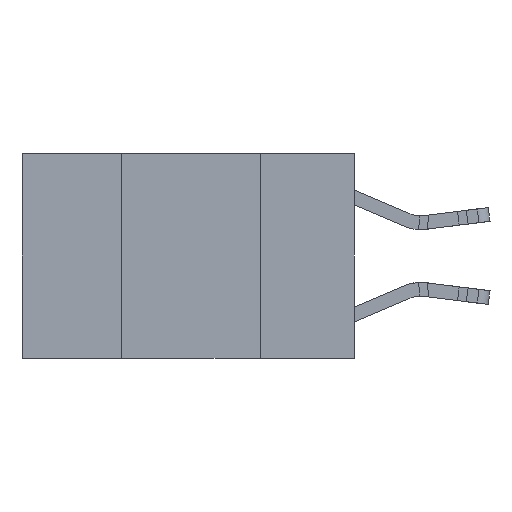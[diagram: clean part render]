
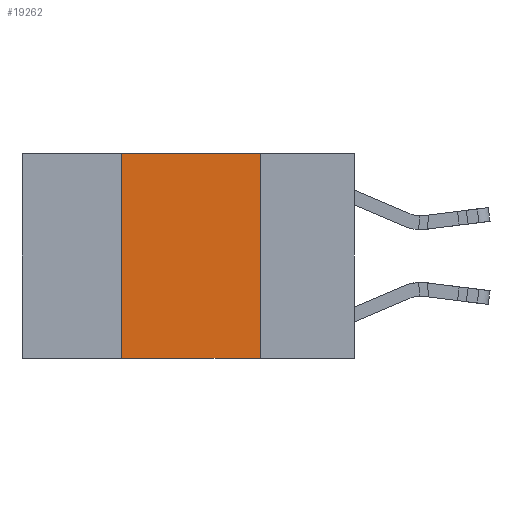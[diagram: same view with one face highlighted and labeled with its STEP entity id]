
A CAD part, left-side view. The second image highlights one B-rep face of the part: STEP entity #19262.
In plain terms, the highlighted planar face has unit normal (-1, 0, 0).
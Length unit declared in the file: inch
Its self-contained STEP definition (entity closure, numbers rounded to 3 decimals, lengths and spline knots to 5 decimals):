
#116 = AXIS2_PLACEMENT_3D ( 'NONE', #16615, #8736, #15577 ) ;
#351 = LINE ( 'NONE', #17271, #19773 ) ;
#1009 = CARTESIAN_POINT ( 'NONE',  ( 0., 0.17, 0. ) ) ;
#2125 = ORIENTED_EDGE ( 'NONE', *, *, #21722, .F. ) ;
#2753 = VERTEX_POINT ( 'NONE', #22281 ) ;
#4189 = PLANE ( 'NONE',  #116 ) ;
#4679 = VECTOR ( 'NONE', #22110, 39.37008 ) ;
#4807 = VERTEX_POINT ( 'NONE', #23476 ) ;
#7535 = CARTESIAN_POINT ( 'NONE',  ( 0., 0.42, 0. ) ) ;
#8060 = LINE ( 'NONE', #24975, #27900 ) ;
#8736 = DIRECTION ( 'NONE',  ( 1., 0., 0. ) ) ;
#9498 = EDGE_CURVE ( 'NONE', #2753, #18724, #351, .T. ) ;
#14685 = ORIENTED_EDGE ( 'NONE', *, *, #21832, .F. ) ;
#15577 = DIRECTION ( 'NONE',  ( 0., 0., -1. ) ) ;
#15973 = FACE_OUTER_BOUND ( 'NONE', #21416, .T. ) ;
#16073 = ORIENTED_EDGE ( 'NONE', *, *, #9498, .F. ) ;
#16615 = CARTESIAN_POINT ( 'NONE',  ( 0., 0.6, 0. ) ) ;
#17271 = CARTESIAN_POINT ( 'NONE',  ( 0., 0.6, 0. ) ) ;
#17430 = DIRECTION ( 'NONE',  ( 0., -1., 0. ) ) ;
#18724 = VERTEX_POINT ( 'NONE', #26451 ) ;
#19262 = ADVANCED_FACE ( 'NONE', ( #15973 ), #4189, .F. ) ;
#19627 = EDGE_CURVE ( 'NONE', #4807, #29416, #8060, .T. ) ;
#19773 = VECTOR ( 'NONE', #17430, 39.37008 ) ;
#19839 = ORIENTED_EDGE ( 'NONE', *, *, #19627, .T. ) ;
#20313 = DIRECTION ( 'NONE',  ( 0., -1., 0. ) ) ;
#21416 = EDGE_LOOP ( 'NONE', ( #14685, #16073, #2125, #19839 ) ) ;
#21722 = EDGE_CURVE ( 'NONE', #4807, #2753, #23677, .T. ) ;
#21832 = EDGE_CURVE ( 'NONE', #18724, #29416, #22724, .T. ) ;
#21965 = DIRECTION ( 'NONE',  ( 0., 0., 1. ) ) ;
#22110 = DIRECTION ( 'NONE',  ( 0., 0., -1. ) ) ;
#22281 = CARTESIAN_POINT ( 'NONE',  ( 0., 0.42, 0. ) ) ;
#22724 = LINE ( 'NONE', #1009, #4679 ) ;
#23476 = CARTESIAN_POINT ( 'NONE',  ( 0., 0.42, -0.37 ) ) ;
#23677 = LINE ( 'NONE', #7535, #25501 ) ;
#24975 = CARTESIAN_POINT ( 'NONE',  ( 0., 0.6, -0.37 ) ) ;
#25501 = VECTOR ( 'NONE', #21965, 39.37008 ) ;
#25806 = CARTESIAN_POINT ( 'NONE',  ( 0., 0.17, -0.37 ) ) ;
#26451 = CARTESIAN_POINT ( 'NONE',  ( 0., 0.17, 0. ) ) ;
#27900 = VECTOR ( 'NONE', #20313, 39.37008 ) ;
#29416 = VERTEX_POINT ( 'NONE', #25806 ) ;
